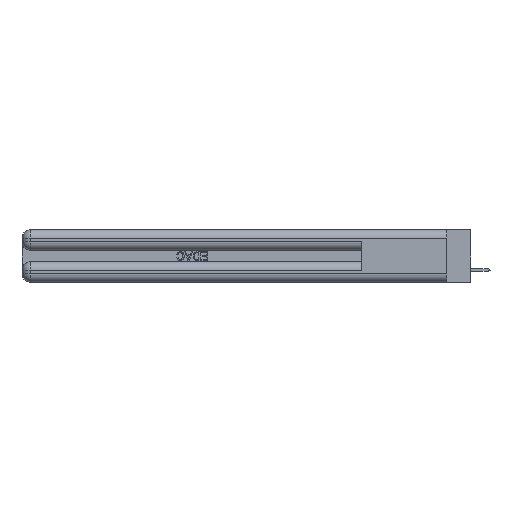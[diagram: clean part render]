
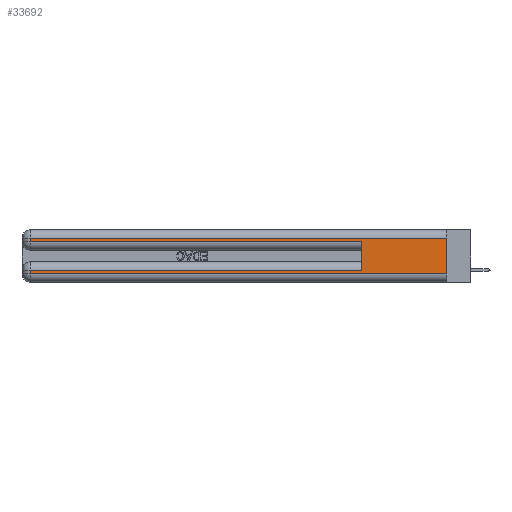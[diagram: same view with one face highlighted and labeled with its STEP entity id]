
A CAD part, left-side view. The second image highlights one B-rep face of the part: STEP entity #33692.
In plain terms, the highlighted planar face has unit normal (-1, 0, 0).
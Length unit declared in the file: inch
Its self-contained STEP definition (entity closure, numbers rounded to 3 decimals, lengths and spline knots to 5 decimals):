
#2037 = LINE ( 'NONE', #23187, #46814 ) ;
#2874 = VECTOR ( 'NONE', #8605, 39.37008 ) ;
#3625 = ORIENTED_EDGE ( 'NONE', *, *, #5584, .F. ) ;
#4181 = VECTOR ( 'NONE', #7109, 39.37008 ) ;
#5115 = LINE ( 'NONE', #39471, #49981 ) ;
#5187 = VERTEX_POINT ( 'NONE', #9756 ) ;
#5387 = DIRECTION ( 'NONE',  ( 0., 0., -1. ) ) ;
#5584 = EDGE_CURVE ( 'NONE', #27656, #42100, #18951, .T. ) ;
#5961 = ORIENTED_EDGE ( 'NONE', *, *, #27611, .T. ) ;
#6427 = VERTEX_POINT ( 'NONE', #47109 ) ;
#6835 = LINE ( 'NONE', #28266, #4181 ) ;
#6942 = DIRECTION ( 'NONE',  ( 0., 1., 0. ) ) ;
#7109 = DIRECTION ( 'NONE',  ( 0., 0., -1. ) ) ;
#8016 = CARTESIAN_POINT ( 'NONE',  ( 0., 2.94, 0.31 ) ) ;
#8505 = FACE_OUTER_BOUND ( 'NONE', #20835, .T. ) ;
#8605 = DIRECTION ( 'NONE',  ( 0., -1., 0. ) ) ;
#8996 = VERTEX_POINT ( 'NONE', #25590 ) ;
#9756 = CARTESIAN_POINT ( 'NONE',  ( 0., 0., 0.06 ) ) ;
#10247 = EDGE_CURVE ( 'NONE', #25020, #5187, #42107, .T. ) ;
#10935 = EDGE_CURVE ( 'NONE', #6427, #5187, #6835, .T. ) ;
#10954 = AXIS2_PLACEMENT_3D ( 'NONE', #24971, #12352, #29108 ) ;
#12352 = DIRECTION ( 'NONE',  ( 1., 0., 0. ) ) ;
#15910 = CARTESIAN_POINT ( 'NONE',  ( 0., 2.94, 0.085 ) ) ;
#17881 = ORIENTED_EDGE ( 'NONE', *, *, #45100, .T. ) ;
#18806 = DIRECTION ( 'NONE',  ( 0., 0., -1. ) ) ;
#18837 = CARTESIAN_POINT ( 'NONE',  ( 0., 2.94, 0.06 ) ) ;
#18951 = LINE ( 'NONE', #23059, #35636 ) ;
#20835 = EDGE_LOOP ( 'NONE', ( #35756, #24512, #17881, #5961, #3625, #26349, #29047, #48692 ) ) ;
#21822 = CARTESIAN_POINT ( 'NONE',  ( 0., 0., 0.085 ) ) ;
#23059 = CARTESIAN_POINT ( 'NONE',  ( 0., 0.6, 0.145 ) ) ;
#23187 = CARTESIAN_POINT ( 'NONE',  ( 0., 2.94, 0.37 ) ) ;
#24512 = ORIENTED_EDGE ( 'NONE', *, *, #52334, .T. ) ;
#24641 = LINE ( 'NONE', #53520, #45683 ) ;
#24971 = CARTESIAN_POINT ( 'NONE',  ( 0., 0., 0.37 ) ) ;
#25020 = VERTEX_POINT ( 'NONE', #18837 ) ;
#25590 = CARTESIAN_POINT ( 'NONE',  ( 0., 2.94, 0.285 ) ) ;
#26349 = ORIENTED_EDGE ( 'NONE', *, *, #49125, .T. ) ;
#27611 = EDGE_CURVE ( 'NONE', #8996, #42100, #24641, .T. ) ;
#27656 = VERTEX_POINT ( 'NONE', #49660 ) ;
#28266 = CARTESIAN_POINT ( 'NONE',  ( 0., 0., 0.37 ) ) ;
#29047 = ORIENTED_EDGE ( 'NONE', *, *, #53587, .T. ) ;
#29108 = DIRECTION ( 'NONE',  ( 0., 0., -1. ) ) ;
#29374 = PLANE ( 'NONE',  #10954 ) ;
#30568 = VECTOR ( 'NONE', #6942, 39.37008 ) ;
#33692 = ADVANCED_FACE ( 'NONE', ( #8505 ), #29374, .F. ) ;
#33857 = CARTESIAN_POINT ( 'NONE',  ( 0., 0., 0.06 ) ) ;
#34554 = CARTESIAN_POINT ( 'NONE',  ( 0., 0.6, 0.285 ) ) ;
#34723 = VECTOR ( 'NONE', #42715, 39.37008 ) ;
#35287 = LINE ( 'NONE', #21822, #34723 ) ;
#35636 = VECTOR ( 'NONE', #47524, 39.37008 ) ;
#35756 = ORIENTED_EDGE ( 'NONE', *, *, #10935, .F. ) ;
#36884 = LINE ( 'NONE', #41556, #30568 ) ;
#39471 = CARTESIAN_POINT ( 'NONE',  ( 0., 2.94, 0.37 ) ) ;
#41148 = DIRECTION ( 'NONE',  ( 0., -1., 0. ) ) ;
#41556 = CARTESIAN_POINT ( 'NONE',  ( 0., 0., 0.31 ) ) ;
#41558 = VERTEX_POINT ( 'NONE', #8016 ) ;
#42100 = VERTEX_POINT ( 'NONE', #34554 ) ;
#42107 = LINE ( 'NONE', #33857, #2874 ) ;
#42715 = DIRECTION ( 'NONE',  ( 0., 1., 0. ) ) ;
#45100 = EDGE_CURVE ( 'NONE', #41558, #8996, #2037, .T. ) ;
#45683 = VECTOR ( 'NONE', #41148, 39.37008 ) ;
#46814 = VECTOR ( 'NONE', #18806, 39.37008 ) ;
#47109 = CARTESIAN_POINT ( 'NONE',  ( 0., 0., 0.31 ) ) ;
#47331 = VERTEX_POINT ( 'NONE', #15910 ) ;
#47524 = DIRECTION ( 'NONE',  ( 0., 0., 1. ) ) ;
#48692 = ORIENTED_EDGE ( 'NONE', *, *, #10247, .T. ) ;
#49125 = EDGE_CURVE ( 'NONE', #27656, #47331, #35287, .T. ) ;
#49660 = CARTESIAN_POINT ( 'NONE',  ( 0., 0.6, 0.085 ) ) ;
#49981 = VECTOR ( 'NONE', #5387, 39.37008 ) ;
#52334 = EDGE_CURVE ( 'NONE', #6427, #41558, #36884, .T. ) ;
#53520 = CARTESIAN_POINT ( 'NONE',  ( 0., 0., 0.285 ) ) ;
#53587 = EDGE_CURVE ( 'NONE', #47331, #25020, #5115, .T. ) ;
